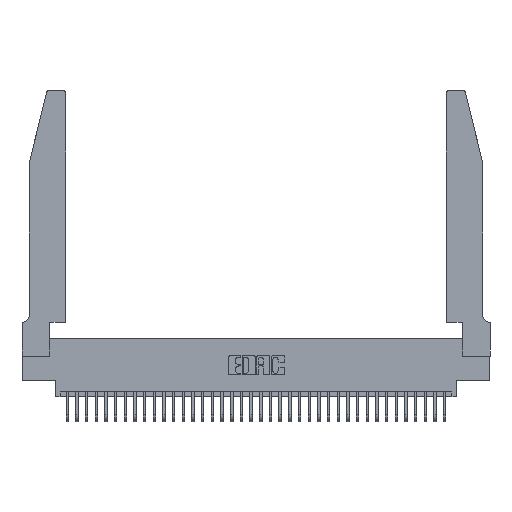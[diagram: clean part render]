
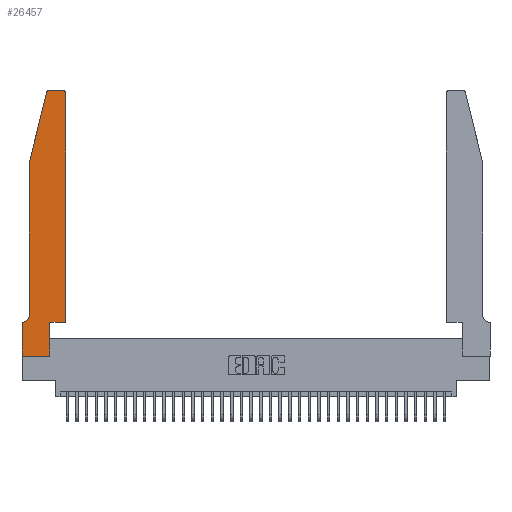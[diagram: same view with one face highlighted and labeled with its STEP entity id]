
A CAD part, top view. The second image highlights one B-rep face of the part: STEP entity #26457.
In plain terms, the highlighted planar face has unit normal (0, 0, 1).
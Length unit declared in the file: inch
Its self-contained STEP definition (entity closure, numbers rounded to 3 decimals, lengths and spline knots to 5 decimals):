
#93 = EDGE_CURVE ( 'NONE', #7713, #4611, #9561, .T. ) ;
#339 = VECTOR ( 'NONE', #610, 39.37008 ) ;
#610 = DIRECTION ( 'NONE',  ( -0.239, -0.971, 0. ) ) ;
#1280 = VERTEX_POINT ( 'NONE', #3944 ) ;
#1415 = CIRCLE ( 'NONE', #10531, 0.03 ) ;
#1674 = DIRECTION ( 'NONE',  ( 0., 0., -1. ) ) ;
#1915 = VERTEX_POINT ( 'NONE', #26698 ) ;
#3193 = CARTESIAN_POINT ( 'NONE',  ( 0.4505, 0.35, 0.37 ) ) ;
#3243 = CARTESIAN_POINT ( 'NONE',  ( 0.284, 2.75, 0.37 ) ) ;
#3520 = VERTEX_POINT ( 'NONE', #7162 ) ;
#3521 = DIRECTION ( 'NONE',  ( 0., -1., 0. ) ) ;
#3944 = CARTESIAN_POINT ( 'NONE',  ( 0.25487, 2.72718, 0.37 ) ) ;
#3961 = EDGE_CURVE ( 'NONE', #1280, #13908, #28660, .T. ) ;
#4015 = VECTOR ( 'NONE', #8329, 39.37008 ) ;
#4342 = EDGE_CURVE ( 'NONE', #8143, #15767, #23174, .T. ) ;
#4611 = VERTEX_POINT ( 'NONE', #14137 ) ;
#4741 = DIRECTION ( 'NONE',  ( 0., -1., 0. ) ) ;
#5103 = EDGE_CURVE ( 'NONE', #15767, #13970, #20984, .T. ) ;
#5395 = PLANE ( 'NONE',  #29602 ) ;
#5912 = CARTESIAN_POINT ( 'NONE',  ( 0.4205, 2.72, 0.37 ) ) ;
#6036 = ORIENTED_EDGE ( 'NONE', *, *, #18856, .T. ) ;
#6117 = DIRECTION ( 'NONE',  ( -1., 0., 0. ) ) ;
#6988 = EDGE_LOOP ( 'NONE', ( #12418, #28661, #7261, #31444, #16724, #32354, #32764, #34855, #12820, #6036, #19944, #20380 ) ) ;
#7162 = CARTESIAN_POINT ( 'NONE',  ( 0.4505, 0.35, 0.37 ) ) ;
#7261 = ORIENTED_EDGE ( 'NONE', *, *, #3961, .T. ) ;
#7309 = DIRECTION ( 'NONE',  ( 0., 0., 1. ) ) ;
#7434 = CARTESIAN_POINT ( 'NONE',  ( 0.4505, 0.35, 0.37 ) ) ;
#7713 = VERTEX_POINT ( 'NONE', #27319 ) ;
#7826 = LINE ( 'NONE', #21146, #21649 ) ;
#8140 = DIRECTION ( 'NONE',  ( 0., 0., 1. ) ) ;
#8143 = VERTEX_POINT ( 'NONE', #15770 ) ;
#8329 = DIRECTION ( 'NONE',  ( -1., 0., 0. ) ) ;
#8656 = DIRECTION ( 'NONE',  ( 1., 0., 0. ) ) ;
#8917 = LINE ( 'NONE', #3193, #27358 ) ;
#9447 = CARTESIAN_POINT ( 'NONE',  ( 0.2865, 0.35, 0.37 ) ) ;
#9561 = LINE ( 'NONE', #29658, #15242 ) ;
#10338 = EDGE_CURVE ( 'NONE', #32317, #25983, #25940, .T. ) ;
#10531 = AXIS2_PLACEMENT_3D ( 'NONE', #23802, #7309, #26496 ) ;
#12418 = ORIENTED_EDGE ( 'NONE', *, *, #10338, .T. ) ;
#12820 = ORIENTED_EDGE ( 'NONE', *, *, #27034, .T. ) ;
#13908 = VERTEX_POINT ( 'NONE', #24699 ) ;
#13970 = VERTEX_POINT ( 'NONE', #30787 ) ;
#14137 = CARTESIAN_POINT ( 'NONE',  ( 0.2865, 0., 0.37 ) ) ;
#14222 = VECTOR ( 'NONE', #3521, 39.37008 ) ;
#14526 = VECTOR ( 'NONE', #6117, 39.37008 ) ;
#14899 = LINE ( 'NONE', #7434, #28511 ) ;
#15242 = VECTOR ( 'NONE', #28135, 39.37008 ) ;
#15515 = AXIS2_PLACEMENT_3D ( 'NONE', #18291, #1674, #21009 ) ;
#15539 = LINE ( 'NONE', #9447, #16416 ) ;
#15767 = VERTEX_POINT ( 'NONE', #27870 ) ;
#15770 = CARTESIAN_POINT ( 'NONE',  ( 0.0755, 0.42, 0.37 ) ) ;
#16414 = CARTESIAN_POINT ( 'NONE',  ( 0., 0.35, 0.37 ) ) ;
#16416 = VECTOR ( 'NONE', #23219, 39.37008 ) ;
#16724 = ORIENTED_EDGE ( 'NONE', *, *, #4342, .T. ) ;
#18291 = CARTESIAN_POINT ( 'NONE',  ( 0.0055, 0.42, 0.37 ) ) ;
#18856 = EDGE_CURVE ( 'NONE', #1915, #3520, #8917, .T. ) ;
#19021 = VERTEX_POINT ( 'NONE', #20458 ) ;
#19944 = ORIENTED_EDGE ( 'NONE', *, *, #20377, .T. ) ;
#20377 = EDGE_CURVE ( 'NONE', #3520, #19021, #14899, .T. ) ;
#20380 = ORIENTED_EDGE ( 'NONE', *, *, #32479, .T. ) ;
#20458 = CARTESIAN_POINT ( 'NONE',  ( 0.4505, 2.72, 0.37 ) ) ;
#20984 = LINE ( 'NONE', #22647, #14526 ) ;
#21009 = DIRECTION ( 'NONE',  ( -1., 0., 0. ) ) ;
#21146 = CARTESIAN_POINT ( 'NONE',  ( 0.0755, 2., 0.37 ) ) ;
#21522 = LINE ( 'NONE', #22838, #14222 ) ;
#21649 = VECTOR ( 'NONE', #4741, 39.37008 ) ;
#22510 = AXIS2_PLACEMENT_3D ( 'NONE', #5912, #25140, #8656 ) ;
#22647 = CARTESIAN_POINT ( 'NONE',  ( 0.0755, 0.35, 0.37 ) ) ;
#22702 = CARTESIAN_POINT ( 'NONE',  ( 0.0755, 2., 0.37 ) ) ;
#22838 = CARTESIAN_POINT ( 'NONE',  ( 0., 0., 0.37 ) ) ;
#23174 = CIRCLE ( 'NONE', #15515, 0.07 ) ;
#23219 = DIRECTION ( 'NONE',  ( 0., 1., 0. ) ) ;
#23802 = CARTESIAN_POINT ( 'NONE',  ( 0.284, 2.72, 0.37 ) ) ;
#23955 = EDGE_CURVE ( 'NONE', #25983, #1280, #1415, .T. ) ;
#24699 = CARTESIAN_POINT ( 'NONE',  ( 0.0755, 2., 0.37 ) ) ;
#24820 = CARTESIAN_POINT ( 'NONE',  ( 0.2605, 2.75, 0.37 ) ) ;
#25140 = DIRECTION ( 'NONE',  ( 0., 0., 1. ) ) ;
#25209 = DIRECTION ( 'NONE',  ( 1., 0., 0. ) ) ;
#25940 = LINE ( 'NONE', #24820, #4015 ) ;
#25983 = VERTEX_POINT ( 'NONE', #3243 ) ;
#26457 = ADVANCED_FACE ( 'NONE', ( #27068 ), #5395, .T. ) ;
#26496 = DIRECTION ( 'NONE',  ( 1., 0., 0. ) ) ;
#26698 = CARTESIAN_POINT ( 'NONE',  ( 0.2865, 0.35, 0.37 ) ) ;
#26974 = CIRCLE ( 'NONE', #22510, 0.03 ) ;
#27034 = EDGE_CURVE ( 'NONE', #4611, #1915, #15539, .T. ) ;
#27068 = FACE_OUTER_BOUND ( 'NONE', #6988, .T. ) ;
#27315 = DIRECTION ( 'NONE',  ( 1., 0., 0. ) ) ;
#27319 = CARTESIAN_POINT ( 'NONE',  ( 0., 0., 0.37 ) ) ;
#27358 = VECTOR ( 'NONE', #25209, 39.37008 ) ;
#27870 = CARTESIAN_POINT ( 'NONE',  ( 0.0055, 0.35, 0.37 ) ) ;
#28135 = DIRECTION ( 'NONE',  ( 1., 0., 0. ) ) ;
#28511 = VECTOR ( 'NONE', #29238, 39.37008 ) ;
#28660 = LINE ( 'NONE', #22702, #339 ) ;
#28661 = ORIENTED_EDGE ( 'NONE', *, *, #23955, .T. ) ;
#29238 = DIRECTION ( 'NONE',  ( 0., 1., 0. ) ) ;
#29563 = EDGE_CURVE ( 'NONE', #13908, #8143, #7826, .T. ) ;
#29602 = AXIS2_PLACEMENT_3D ( 'NONE', #16414, #8140, #27315 ) ;
#29658 = CARTESIAN_POINT ( 'NONE',  ( 0., 0., 0.37 ) ) ;
#29733 = CARTESIAN_POINT ( 'NONE',  ( 0.4205, 2.75, 0.37 ) ) ;
#30787 = CARTESIAN_POINT ( 'NONE',  ( 0., 0.35, 0.37 ) ) ;
#31444 = ORIENTED_EDGE ( 'NONE', *, *, #29563, .T. ) ;
#31947 = EDGE_CURVE ( 'NONE', #13970, #7713, #21522, .T. ) ;
#32317 = VERTEX_POINT ( 'NONE', #29733 ) ;
#32354 = ORIENTED_EDGE ( 'NONE', *, *, #5103, .T. ) ;
#32479 = EDGE_CURVE ( 'NONE', #19021, #32317, #26974, .T. ) ;
#32764 = ORIENTED_EDGE ( 'NONE', *, *, #31947, .T. ) ;
#34855 = ORIENTED_EDGE ( 'NONE', *, *, #93, .T. ) ;
